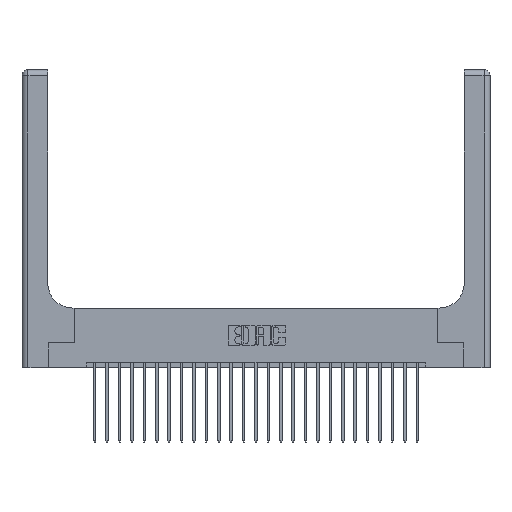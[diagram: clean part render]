
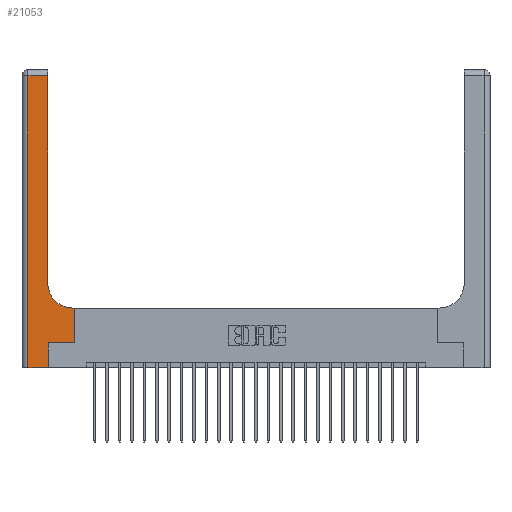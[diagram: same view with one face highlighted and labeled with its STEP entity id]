
A CAD part, top view. The second image highlights one B-rep face of the part: STEP entity #21053.
In plain terms, the highlighted planar face has unit normal (0, 0, 1).
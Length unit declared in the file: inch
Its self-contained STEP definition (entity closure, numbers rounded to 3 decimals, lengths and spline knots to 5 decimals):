
#636 = AXIS2_PLACEMENT_3D ( 'NONE', #17745, #15704, #6184 ) ;
#1415 = LINE ( 'NONE', #10779, #15814 ) ;
#1723 = VERTEX_POINT ( 'NONE', #5685 ) ;
#2266 = CARTESIAN_POINT ( 'NONE',  ( 0.06, 0., 0.37 ) ) ;
#2333 = CARTESIAN_POINT ( 'NONE',  ( 0.265, 0.25, 0.37 ) ) ;
#2339 = AXIS2_PLACEMENT_3D ( 'NONE', #3263, #11095, #3395 ) ;
#2340 = DIRECTION ( 'NONE',  ( -1., 0., 0. ) ) ;
#2902 = VERTEX_POINT ( 'NONE', #11105 ) ;
#2996 = VECTOR ( 'NONE', #16049, 39.37008 ) ;
#3192 = EDGE_CURVE ( 'NONE', #9720, #3868, #5951, .T. ) ;
#3263 = CARTESIAN_POINT ( 'NONE',  ( 0., 3., 0.37 ) ) ;
#3395 = DIRECTION ( 'NONE',  ( -1., 0., 0. ) ) ;
#3510 = CARTESIAN_POINT ( 'NONE',  ( 0.528, 0.25, 0.37 ) ) ;
#3868 = VERTEX_POINT ( 'NONE', #12458 ) ;
#4123 = LINE ( 'NONE', #17730, #22711 ) ;
#4342 = EDGE_CURVE ( 'NONE', #13158, #22212, #11467, .T. ) ;
#5125 = CARTESIAN_POINT ( 'NONE',  ( 0.06, 3., 0.37 ) ) ;
#5452 = DIRECTION ( 'NONE',  ( 0., 1., 0. ) ) ;
#5685 = CARTESIAN_POINT ( 'NONE',  ( 0.265, 0.25, 0.37 ) ) ;
#5951 = CIRCLE ( 'NONE', #636, 0.25 ) ;
#5960 = ORIENTED_EDGE ( 'NONE', *, *, #19658, .T. ) ;
#6184 = DIRECTION ( 'NONE',  ( 1., 0., 0. ) ) ;
#6960 = CARTESIAN_POINT ( 'NONE',  ( 0.51, 0.6, 0.37 ) ) ;
#7073 = ORIENTED_EDGE ( 'NONE', *, *, #15100, .T. ) ;
#7208 = ORIENTED_EDGE ( 'NONE', *, *, #21803, .T. ) ;
#7220 = LINE ( 'NONE', #18624, #10496 ) ;
#7433 = DIRECTION ( 'NONE',  ( 0., -1., 0. ) ) ;
#7440 = ORIENTED_EDGE ( 'NONE', *, *, #3192, .T. ) ;
#8300 = VECTOR ( 'NONE', #17815, 39.37008 ) ;
#9720 = VERTEX_POINT ( 'NONE', #6960 ) ;
#10496 = VECTOR ( 'NONE', #16841, 39.37008 ) ;
#10779 = CARTESIAN_POINT ( 'NONE',  ( 0., 0., 0.37 ) ) ;
#10969 = EDGE_CURVE ( 'NONE', #2902, #23971, #7220, .T. ) ;
#11095 = DIRECTION ( 'NONE',  ( 0., 0., -1. ) ) ;
#11105 = CARTESIAN_POINT ( 'NONE',  ( 0.26, 2.94, 0.37 ) ) ;
#11174 = CARTESIAN_POINT ( 'NONE',  ( 0.265, 0., 0.37 ) ) ;
#11467 = LINE ( 'NONE', #3510, #8300 ) ;
#12236 = CARTESIAN_POINT ( 'NONE',  ( 0.06, 2.94, 0.37 ) ) ;
#12458 = CARTESIAN_POINT ( 'NONE',  ( 0.26, 0.85, 0.37 ) ) ;
#13158 = VERTEX_POINT ( 'NONE', #21067 ) ;
#13167 = LINE ( 'NONE', #21205, #18998 ) ;
#14014 = VECTOR ( 'NONE', #20237, 39.37008 ) ;
#14085 = VERTEX_POINT ( 'NONE', #2266 ) ;
#14225 = VECTOR ( 'NONE', #7433, 39.37008 ) ;
#15100 = EDGE_CURVE ( 'NONE', #22916, #1723, #20976, .T. ) ;
#15704 = DIRECTION ( 'NONE',  ( 0., 0., -1. ) ) ;
#15814 = VECTOR ( 'NONE', #21002, 39.37008 ) ;
#16049 = DIRECTION ( 'NONE',  ( 1., 0., 0. ) ) ;
#16127 = ORIENTED_EDGE ( 'NONE', *, *, #10969, .T. ) ;
#16131 = ORIENTED_EDGE ( 'NONE', *, *, #22919, .T. ) ;
#16312 = ORIENTED_EDGE ( 'NONE', *, *, #16712, .T. ) ;
#16712 = EDGE_CURVE ( 'NONE', #1723, #13158, #18454, .T. ) ;
#16841 = DIRECTION ( 'NONE',  ( -1., 0., 0. ) ) ;
#17182 = LINE ( 'NONE', #5125, #14225 ) ;
#17271 = CARTESIAN_POINT ( 'NONE',  ( 0.528, 0.6, 0.37 ) ) ;
#17730 = CARTESIAN_POINT ( 'NONE',  ( 0.26, 0.6, 0.37 ) ) ;
#17745 = CARTESIAN_POINT ( 'NONE',  ( 0.51, 0.85, 0.37 ) ) ;
#17800 = EDGE_CURVE ( 'NONE', #3868, #2902, #13167, .T. ) ;
#17815 = DIRECTION ( 'NONE',  ( 0., 1., 0. ) ) ;
#18454 = LINE ( 'NONE', #2333, #2996 ) ;
#18624 = CARTESIAN_POINT ( 'NONE',  ( 0., 2.94, 0.37 ) ) ;
#18998 = VECTOR ( 'NONE', #5452, 39.37008 ) ;
#19658 = EDGE_CURVE ( 'NONE', #22212, #9720, #4123, .T. ) ;
#20237 = DIRECTION ( 'NONE',  ( 0., 1., 0. ) ) ;
#20796 = FACE_OUTER_BOUND ( 'NONE', #21292, .T. ) ;
#20918 = ORIENTED_EDGE ( 'NONE', *, *, #4342, .T. ) ;
#20922 = PLANE ( 'NONE',  #2339 ) ;
#20976 = LINE ( 'NONE', #24690, #14014 ) ;
#21002 = DIRECTION ( 'NONE',  ( 1., 0., 0. ) ) ;
#21053 = ADVANCED_FACE ( 'NONE', ( #20796 ), #20922, .F. ) ;
#21067 = CARTESIAN_POINT ( 'NONE',  ( 0.528, 0.25, 0.37 ) ) ;
#21205 = CARTESIAN_POINT ( 'NONE',  ( 0.26, 3., 0.37 ) ) ;
#21292 = EDGE_LOOP ( 'NONE', ( #21316, #16127, #16131, #7208, #7073, #16312, #20918, #5960, #7440 ) ) ;
#21316 = ORIENTED_EDGE ( 'NONE', *, *, #17800, .T. ) ;
#21803 = EDGE_CURVE ( 'NONE', #14085, #22916, #1415, .T. ) ;
#22212 = VERTEX_POINT ( 'NONE', #17271 ) ;
#22711 = VECTOR ( 'NONE', #2340, 39.37008 ) ;
#22916 = VERTEX_POINT ( 'NONE', #11174 ) ;
#22919 = EDGE_CURVE ( 'NONE', #23971, #14085, #17182, .T. ) ;
#23971 = VERTEX_POINT ( 'NONE', #12236 ) ;
#24690 = CARTESIAN_POINT ( 'NONE',  ( 0.265, 0., 0.37 ) ) ;
